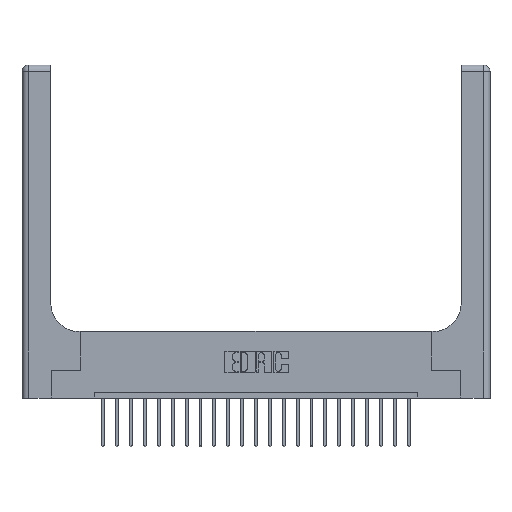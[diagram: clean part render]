
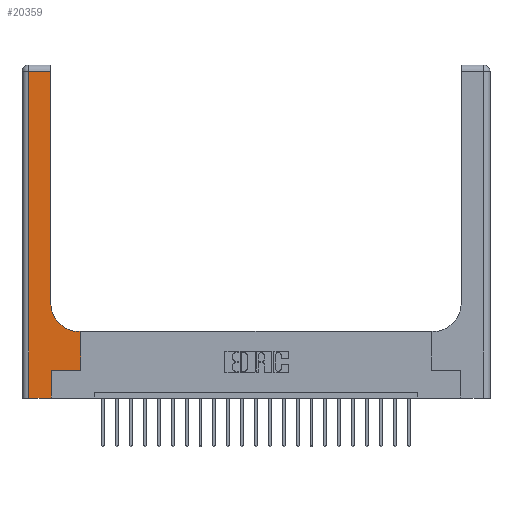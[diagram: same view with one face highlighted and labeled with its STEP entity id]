
A CAD part, top view. The second image highlights one B-rep face of the part: STEP entity #20359.
In plain terms, the highlighted planar face has unit normal (0, 0, 1).
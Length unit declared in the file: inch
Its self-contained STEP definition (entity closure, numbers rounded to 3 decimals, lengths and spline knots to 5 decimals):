
#30 = EDGE_CURVE ( 'NONE', #11368, #15452, #3983, .T. ) ;
#167 = LINE ( 'NONE', #4300, #8164 ) ;
#233 = DIRECTION ( 'NONE',  ( 0., 0., -1. ) ) ;
#800 = CARTESIAN_POINT ( 'NONE',  ( 0.265, 0.25, 0.37 ) ) ;
#813 = LINE ( 'NONE', #4526, #3513 ) ;
#1281 = EDGE_CURVE ( 'NONE', #19016, #11368, #167, .T. ) ;
#1330 = CARTESIAN_POINT ( 'NONE',  ( 0.06, 0., 0.37 ) ) ;
#1340 = DIRECTION ( 'NONE',  ( 0., -1., 0. ) ) ;
#1387 = EDGE_CURVE ( 'NONE', #2250, #11920, #18816, .T. ) ;
#1696 = CARTESIAN_POINT ( 'NONE',  ( 0.265, 0., 0.37 ) ) ;
#1868 = DIRECTION ( 'NONE',  ( 1., 0., 0. ) ) ;
#2250 = VERTEX_POINT ( 'NONE', #10181 ) ;
#2411 = EDGE_CURVE ( 'NONE', #16462, #7042, #9340, .T. ) ;
#3070 = CARTESIAN_POINT ( 'NONE',  ( 0.528, 0.25, 0.37 ) ) ;
#3358 = ORIENTED_EDGE ( 'NONE', *, *, #5032, .T. ) ;
#3513 = VECTOR ( 'NONE', #6239, 39.37008 ) ;
#3911 = VECTOR ( 'NONE', #11187, 39.37008 ) ;
#3946 = PLANE ( 'NONE',  #5845 ) ;
#3983 = LINE ( 'NONE', #9475, #4525 ) ;
#4130 = CARTESIAN_POINT ( 'NONE',  ( 0., 0., 0.37 ) ) ;
#4300 = CARTESIAN_POINT ( 'NONE',  ( 0.26, 3., 0.37 ) ) ;
#4462 = DIRECTION ( 'NONE',  ( 0., 1., 0. ) ) ;
#4525 = VECTOR ( 'NONE', #7582, 39.37008 ) ;
#4526 = CARTESIAN_POINT ( 'NONE',  ( 0.26, 0.6, 0.37 ) ) ;
#4917 = ORIENTED_EDGE ( 'NONE', *, *, #1281, .T. ) ;
#5032 = EDGE_CURVE ( 'NONE', #11920, #19014, #813, .T. ) ;
#5797 = DIRECTION ( 'NONE',  ( 0., 0., -1. ) ) ;
#5845 = AXIS2_PLACEMENT_3D ( 'NONE', #14426, #5797, #12497 ) ;
#6239 = DIRECTION ( 'NONE',  ( -1., 0., 0. ) ) ;
#6449 = EDGE_LOOP ( 'NONE', ( #4917, #16495, #16646, #19297, #15412, #16771, #8733, #3358, #18757 ) ) ;
#6696 = CIRCLE ( 'NONE', #18792, 0.25 ) ;
#7042 = VERTEX_POINT ( 'NONE', #1696 ) ;
#7582 = DIRECTION ( 'NONE',  ( -1., 0., 0. ) ) ;
#8000 = CARTESIAN_POINT ( 'NONE',  ( 0.26, 2.94, 0.37 ) ) ;
#8164 = VECTOR ( 'NONE', #4462, 39.37008 ) ;
#8167 = CARTESIAN_POINT ( 'NONE',  ( 0.26, 0.85, 0.37 ) ) ;
#8733 = ORIENTED_EDGE ( 'NONE', *, *, #1387, .T. ) ;
#9340 = LINE ( 'NONE', #4130, #16794 ) ;
#9475 = CARTESIAN_POINT ( 'NONE',  ( 0., 2.94, 0.37 ) ) ;
#10181 = CARTESIAN_POINT ( 'NONE',  ( 0.528, 0.25, 0.37 ) ) ;
#10333 = VECTOR ( 'NONE', #18452, 39.37008 ) ;
#10979 = CARTESIAN_POINT ( 'NONE',  ( 0.265, 0.25, 0.37 ) ) ;
#10984 = DIRECTION ( 'NONE',  ( 1., 0., 0. ) ) ;
#11187 = DIRECTION ( 'NONE',  ( 1., 0., 0. ) ) ;
#11368 = VERTEX_POINT ( 'NONE', #8000 ) ;
#11490 = DIRECTION ( 'NONE',  ( 0., 1., 0. ) ) ;
#11554 = CARTESIAN_POINT ( 'NONE',  ( 0.265, 0., 0.37 ) ) ;
#11803 = VECTOR ( 'NONE', #1340, 39.37008 ) ;
#11920 = VERTEX_POINT ( 'NONE', #18468 ) ;
#12005 = CARTESIAN_POINT ( 'NONE',  ( 0.51, 0.85, 0.37 ) ) ;
#12011 = CARTESIAN_POINT ( 'NONE',  ( 0.06, 2.94, 0.37 ) ) ;
#12497 = DIRECTION ( 'NONE',  ( -1., 0., 0. ) ) ;
#12590 = EDGE_CURVE ( 'NONE', #15452, #16462, #18454, .T. ) ;
#12976 = LINE ( 'NONE', #800, #3911 ) ;
#13032 = LINE ( 'NONE', #11554, #14873 ) ;
#13338 = CARTESIAN_POINT ( 'NONE',  ( 0.06, 3., 0.37 ) ) ;
#13536 = VERTEX_POINT ( 'NONE', #10979 ) ;
#14426 = CARTESIAN_POINT ( 'NONE',  ( 0., 3., 0.37 ) ) ;
#14873 = VECTOR ( 'NONE', #11490, 39.37008 ) ;
#15002 = CARTESIAN_POINT ( 'NONE',  ( 0.51, 0.6, 0.37 ) ) ;
#15412 = ORIENTED_EDGE ( 'NONE', *, *, #15788, .T. ) ;
#15452 = VERTEX_POINT ( 'NONE', #12011 ) ;
#15651 = FACE_OUTER_BOUND ( 'NONE', #6449, .T. ) ;
#15788 = EDGE_CURVE ( 'NONE', #7042, #13536, #13032, .T. ) ;
#16462 = VERTEX_POINT ( 'NONE', #1330 ) ;
#16495 = ORIENTED_EDGE ( 'NONE', *, *, #30, .T. ) ;
#16646 = ORIENTED_EDGE ( 'NONE', *, *, #12590, .T. ) ;
#16771 = ORIENTED_EDGE ( 'NONE', *, *, #21177, .T. ) ;
#16794 = VECTOR ( 'NONE', #10984, 39.37008 ) ;
#17215 = EDGE_CURVE ( 'NONE', #19014, #19016, #6696, .T. ) ;
#18452 = DIRECTION ( 'NONE',  ( 0., 1., 0. ) ) ;
#18454 = LINE ( 'NONE', #13338, #11803 ) ;
#18468 = CARTESIAN_POINT ( 'NONE',  ( 0.528, 0.6, 0.37 ) ) ;
#18757 = ORIENTED_EDGE ( 'NONE', *, *, #17215, .T. ) ;
#18792 = AXIS2_PLACEMENT_3D ( 'NONE', #12005, #233, #1868 ) ;
#18816 = LINE ( 'NONE', #3070, #10333 ) ;
#19014 = VERTEX_POINT ( 'NONE', #15002 ) ;
#19016 = VERTEX_POINT ( 'NONE', #8167 ) ;
#19297 = ORIENTED_EDGE ( 'NONE', *, *, #2411, .T. ) ;
#20359 = ADVANCED_FACE ( 'NONE', ( #15651 ), #3946, .F. ) ;
#21177 = EDGE_CURVE ( 'NONE', #13536, #2250, #12976, .T. ) ;
